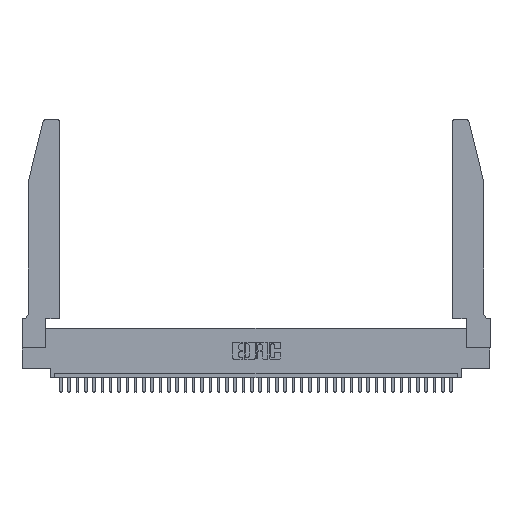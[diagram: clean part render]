
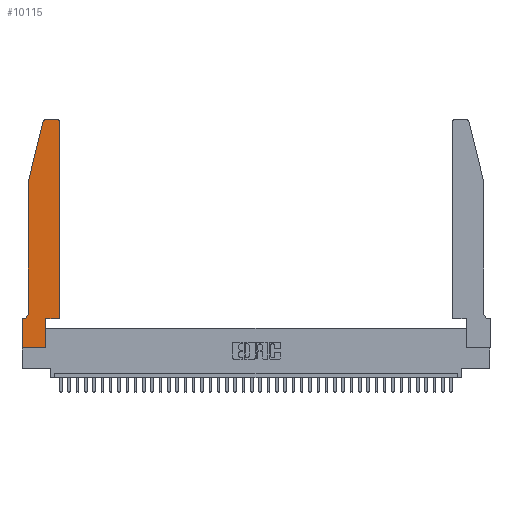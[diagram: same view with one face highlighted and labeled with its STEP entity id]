
A CAD part, top view. The second image highlights one B-rep face of the part: STEP entity #10115.
In plain terms, the highlighted planar face has unit normal (0, 0, 1).
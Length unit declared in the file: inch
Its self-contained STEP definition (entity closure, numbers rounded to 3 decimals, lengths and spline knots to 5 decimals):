
#1239 = VERTEX_POINT ( 'NONE', #10742 ) ;
#1473 = DIRECTION ( 'NONE',  ( 0., -1., 0. ) ) ;
#1779 = VECTOR ( 'NONE', #4192, 39.37008 ) ;
#2176 = CARTESIAN_POINT ( 'NONE',  ( 0., 0., 0.37 ) ) ;
#2404 = VECTOR ( 'NONE', #11029, 39.37008 ) ;
#2810 = ORIENTED_EDGE ( 'NONE', *, *, #28030, .T. ) ;
#3065 = EDGE_CURVE ( 'NONE', #5810, #14527, #32845, .T. ) ;
#3134 = DIRECTION ( 'NONE',  ( 0., 0., 1. ) ) ;
#3641 = EDGE_CURVE ( 'NONE', #9238, #12069, #34242, .T. ) ;
#4192 = DIRECTION ( 'NONE',  ( -1., 0., 0. ) ) ;
#5063 = VERTEX_POINT ( 'NONE', #29646 ) ;
#5810 = VERTEX_POINT ( 'NONE', #23155 ) ;
#6445 = ORIENTED_EDGE ( 'NONE', *, *, #24666, .T. ) ;
#6806 = CARTESIAN_POINT ( 'NONE',  ( 0.4205, 2.75, 0.37 ) ) ;
#6881 = EDGE_CURVE ( 'NONE', #30464, #20514, #11206, .T. ) ;
#6956 = DIRECTION ( 'NONE',  ( -0.239, -0.971, 0. ) ) ;
#7835 = AXIS2_PLACEMENT_3D ( 'NONE', #25544, #10037, #16002 ) ;
#8700 = CARTESIAN_POINT ( 'NONE',  ( 0.4505, 0.35, 0.37 ) ) ;
#8786 = LINE ( 'NONE', #38460, #33144 ) ;
#9138 = PLANE ( 'NONE',  #7835 ) ;
#9238 = VERTEX_POINT ( 'NONE', #38781 ) ;
#9437 = VECTOR ( 'NONE', #1473, 39.37008 ) ;
#10037 = DIRECTION ( 'NONE',  ( 0., 0., 1. ) ) ;
#10115 = ADVANCED_FACE ( 'NONE', ( #19142 ), #9138, .T. ) ;
#10575 = DIRECTION ( 'NONE',  ( 1., 0., 0. ) ) ;
#10627 = CARTESIAN_POINT ( 'NONE',  ( 0.284, 2.72, 0.37 ) ) ;
#10742 = CARTESIAN_POINT ( 'NONE',  ( 0.0755, 2., 0.37 ) ) ;
#11029 = DIRECTION ( 'NONE',  ( 0., 1., 0. ) ) ;
#11206 = LINE ( 'NONE', #36854, #28692 ) ;
#11412 = EDGE_CURVE ( 'NONE', #5063, #9238, #26125, .T. ) ;
#11668 = EDGE_CURVE ( 'NONE', #22388, #17490, #8786, .T. ) ;
#12069 = VERTEX_POINT ( 'NONE', #13540 ) ;
#12163 = VECTOR ( 'NONE', #19986, 39.37008 ) ;
#12264 = ORIENTED_EDGE ( 'NONE', *, *, #24835, .T. ) ;
#13147 = DIRECTION ( 'NONE',  ( 1., 0., 0. ) ) ;
#13225 = ORIENTED_EDGE ( 'NONE', *, *, #11412, .T. ) ;
#13283 = ORIENTED_EDGE ( 'NONE', *, *, #32123, .T. ) ;
#13390 = ORIENTED_EDGE ( 'NONE', *, *, #6881, .T. ) ;
#13505 = DIRECTION ( 'NONE',  ( -1., 0., 0. ) ) ;
#13540 = CARTESIAN_POINT ( 'NONE',  ( 0.2865, 0., 0.37 ) ) ;
#13871 = CIRCLE ( 'NONE', #17766, 0.03 ) ;
#14527 = VERTEX_POINT ( 'NONE', #25790 ) ;
#15793 = CARTESIAN_POINT ( 'NONE',  ( 0.0755, 2., 0.37 ) ) ;
#15864 = ORIENTED_EDGE ( 'NONE', *, *, #3065, .T. ) ;
#16002 = DIRECTION ( 'NONE',  ( 1., 0., 0. ) ) ;
#16130 = DIRECTION ( 'NONE',  ( 1., 0., 0. ) ) ;
#16173 = LINE ( 'NONE', #16286, #9437 ) ;
#16286 = CARTESIAN_POINT ( 'NONE',  ( 0.0755, 2., 0.37 ) ) ;
#16695 = CARTESIAN_POINT ( 'NONE',  ( 0.2865, 0.35, 0.37 ) ) ;
#17490 = VERTEX_POINT ( 'NONE', #28232 ) ;
#17766 = AXIS2_PLACEMENT_3D ( 'NONE', #34784, #31796, #16130 ) ;
#18391 = VERTEX_POINT ( 'NONE', #39605 ) ;
#18603 = CARTESIAN_POINT ( 'NONE',  ( 0.25487, 2.72718, 0.37 ) ) ;
#18939 = LINE ( 'NONE', #16695, #12163 ) ;
#19142 = FACE_OUTER_BOUND ( 'NONE', #23663, .T. ) ;
#19784 = DIRECTION ( 'NONE',  ( 0., -1., 0. ) ) ;
#19820 = EDGE_CURVE ( 'NONE', #1239, #5810, #16173, .T. ) ;
#19986 = DIRECTION ( 'NONE',  ( 0., 1., 0. ) ) ;
#20514 = VERTEX_POINT ( 'NONE', #29059 ) ;
#20668 = VERTEX_POINT ( 'NONE', #18603 ) ;
#21312 = LINE ( 'NONE', #22829, #1779 ) ;
#21674 = VECTOR ( 'NONE', #6956, 39.37008 ) ;
#21977 = EDGE_CURVE ( 'NONE', #12069, #22388, #18939, .T. ) ;
#22388 = VERTEX_POINT ( 'NONE', #34962 ) ;
#22829 = CARTESIAN_POINT ( 'NONE',  ( 0.0755, 0.35, 0.37 ) ) ;
#23155 = CARTESIAN_POINT ( 'NONE',  ( 0.0755, 0.42, 0.37 ) ) ;
#23663 = EDGE_LOOP ( 'NONE', ( #13390, #6445, #12264, #26743, #15864, #13283, #13225, #24003, #35482, #35972, #2810, #37634 ) ) ;
#24003 = ORIENTED_EDGE ( 'NONE', *, *, #3641, .T. ) ;
#24666 = EDGE_CURVE ( 'NONE', #20514, #20668, #28416, .T. ) ;
#24835 = EDGE_CURVE ( 'NONE', #20668, #1239, #32862, .T. ) ;
#24948 = EDGE_CURVE ( 'NONE', #18391, #30464, #13871, .T. ) ;
#25544 = CARTESIAN_POINT ( 'NONE',  ( 0., 0.35, 0.37 ) ) ;
#25790 = CARTESIAN_POINT ( 'NONE',  ( 0.0055, 0.35, 0.37 ) ) ;
#25981 = VECTOR ( 'NONE', #13147, 39.37008 ) ;
#26125 = LINE ( 'NONE', #39554, #36862 ) ;
#26743 = ORIENTED_EDGE ( 'NONE', *, *, #19820, .T. ) ;
#28030 = EDGE_CURVE ( 'NONE', #17490, #18391, #29192, .T. ) ;
#28232 = CARTESIAN_POINT ( 'NONE',  ( 0.4505, 0.35, 0.37 ) ) ;
#28416 = CIRCLE ( 'NONE', #39951, 0.03 ) ;
#28692 = VECTOR ( 'NONE', #30500, 39.37008 ) ;
#29059 = CARTESIAN_POINT ( 'NONE',  ( 0.284, 2.75, 0.37 ) ) ;
#29192 = LINE ( 'NONE', #8700, #2404 ) ;
#29646 = CARTESIAN_POINT ( 'NONE',  ( 0., 0.35, 0.37 ) ) ;
#29858 = AXIS2_PLACEMENT_3D ( 'NONE', #32578, #38699, #13505 ) ;
#30464 = VERTEX_POINT ( 'NONE', #6806 ) ;
#30500 = DIRECTION ( 'NONE',  ( -1., 0., 0. ) ) ;
#31796 = DIRECTION ( 'NONE',  ( 0., 0., 1. ) ) ;
#32123 = EDGE_CURVE ( 'NONE', #14527, #5063, #21312, .T. ) ;
#32578 = CARTESIAN_POINT ( 'NONE',  ( 0.0055, 0.42, 0.37 ) ) ;
#32845 = CIRCLE ( 'NONE', #29858, 0.07 ) ;
#32862 = LINE ( 'NONE', #15793, #21674 ) ;
#33144 = VECTOR ( 'NONE', #10575, 39.37008 ) ;
#34242 = LINE ( 'NONE', #2176, #25981 ) ;
#34784 = CARTESIAN_POINT ( 'NONE',  ( 0.4205, 2.72, 0.37 ) ) ;
#34962 = CARTESIAN_POINT ( 'NONE',  ( 0.2865, 0.35, 0.37 ) ) ;
#35482 = ORIENTED_EDGE ( 'NONE', *, *, #21977, .T. ) ;
#35972 = ORIENTED_EDGE ( 'NONE', *, *, #11668, .T. ) ;
#36854 = CARTESIAN_POINT ( 'NONE',  ( 0.2605, 2.75, 0.37 ) ) ;
#36862 = VECTOR ( 'NONE', #19784, 39.37008 ) ;
#37634 = ORIENTED_EDGE ( 'NONE', *, *, #24948, .T. ) ;
#38460 = CARTESIAN_POINT ( 'NONE',  ( 0.4505, 0.35, 0.37 ) ) ;
#38699 = DIRECTION ( 'NONE',  ( 0., 0., -1. ) ) ;
#38781 = CARTESIAN_POINT ( 'NONE',  ( 0., 0., 0.37 ) ) ;
#39071 = DIRECTION ( 'NONE',  ( 1., 0., 0. ) ) ;
#39554 = CARTESIAN_POINT ( 'NONE',  ( 0., 0., 0.37 ) ) ;
#39605 = CARTESIAN_POINT ( 'NONE',  ( 0.4505, 2.72, 0.37 ) ) ;
#39951 = AXIS2_PLACEMENT_3D ( 'NONE', #10627, #3134, #39071 ) ;
